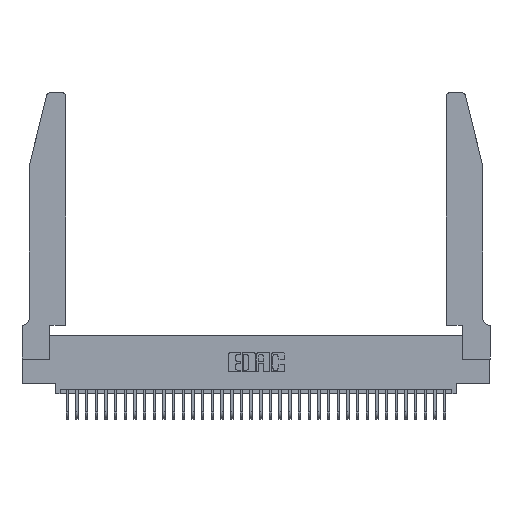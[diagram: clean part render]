
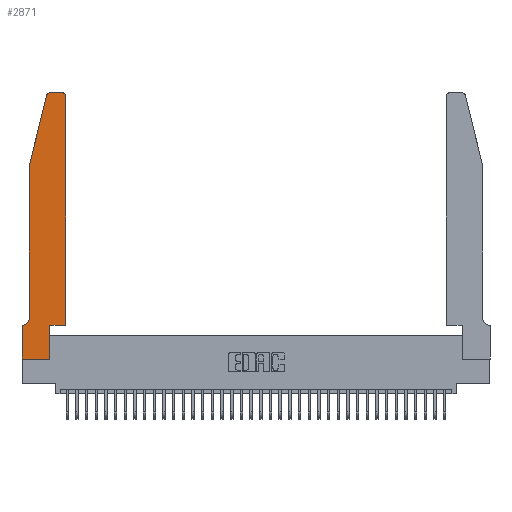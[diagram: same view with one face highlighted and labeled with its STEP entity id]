
A CAD part, top view. The second image highlights one B-rep face of the part: STEP entity #2871.
In plain terms, the highlighted planar face has unit normal (0, 0, 1).
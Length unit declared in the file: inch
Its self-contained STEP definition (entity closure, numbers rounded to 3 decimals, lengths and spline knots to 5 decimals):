
#1622 = EDGE_CURVE ( 'NONE', #17877, #11990, #17657, .T. ) ;
#1650 = CARTESIAN_POINT ( 'NONE',  ( 0., 0., 0.37 ) ) ;
#1932 = AXIS2_PLACEMENT_3D ( 'NONE', #25203, #11675, #30626 ) ;
#2622 = CARTESIAN_POINT ( 'NONE',  ( 0.0055, 0.35, 0.37 ) ) ;
#2848 = AXIS2_PLACEMENT_3D ( 'NONE', #14310, #33249, #17055 ) ;
#2871 = ADVANCED_FACE ( 'NONE', ( #5608 ), #8942, .T. ) ;
#3245 = ORIENTED_EDGE ( 'NONE', *, *, #9922, .T. ) ;
#4492 = ORIENTED_EDGE ( 'NONE', *, *, #1622, .T. ) ;
#5138 = EDGE_CURVE ( 'NONE', #32559, #6090, #13553, .T. ) ;
#5183 = VERTEX_POINT ( 'NONE', #2622 ) ;
#5518 = CARTESIAN_POINT ( 'NONE',  ( 0., 0., 0.37 ) ) ;
#5608 = FACE_OUTER_BOUND ( 'NONE', #26734, .T. ) ;
#6090 = VERTEX_POINT ( 'NONE', #24493 ) ;
#6145 = VERTEX_POINT ( 'NONE', #8455 ) ;
#6297 = VECTOR ( 'NONE', #32265, 39.37008 ) ;
#7257 = DIRECTION ( 'NONE',  ( 0., -1., 0. ) ) ;
#7397 = CARTESIAN_POINT ( 'NONE',  ( 0.4205, 2.72, 0.37 ) ) ;
#7553 = CARTESIAN_POINT ( 'NONE',  ( 0.2605, 2.75, 0.37 ) ) ;
#7961 = ORIENTED_EDGE ( 'NONE', *, *, #5138, .T. ) ;
#8039 = ORIENTED_EDGE ( 'NONE', *, *, #30061, .T. ) ;
#8318 = ORIENTED_EDGE ( 'NONE', *, *, #28478, .T. ) ;
#8455 = CARTESIAN_POINT ( 'NONE',  ( 0., 0.35, 0.37 ) ) ;
#8689 = CARTESIAN_POINT ( 'NONE',  ( 0.0755, 2., 0.37 ) ) ;
#8726 = ORIENTED_EDGE ( 'NONE', *, *, #23400, .T. ) ;
#8939 = ORIENTED_EDGE ( 'NONE', *, *, #12916, .T. ) ;
#8942 = PLANE ( 'NONE',  #1932 ) ;
#9538 = CARTESIAN_POINT ( 'NONE',  ( 0.2865, 0.35, 0.37 ) ) ;
#9587 = VECTOR ( 'NONE', #21124, 39.37008 ) ;
#9773 = DIRECTION ( 'NONE',  ( 0., 0., 1. ) ) ;
#9900 = VECTOR ( 'NONE', #33381, 39.37008 ) ;
#9922 = EDGE_CURVE ( 'NONE', #26077, #32559, #25986, .T. ) ;
#9949 = EDGE_CURVE ( 'NONE', #32544, #17877, #25138, .T. ) ;
#10133 = DIRECTION ( 'NONE',  ( 1., 0., 0. ) ) ;
#11533 = VECTOR ( 'NONE', #32969, 39.37008 ) ;
#11675 = DIRECTION ( 'NONE',  ( 0., 0., 1. ) ) ;
#11715 = CARTESIAN_POINT ( 'NONE',  ( 0.0755, 2., 0.37 ) ) ;
#11990 = VERTEX_POINT ( 'NONE', #26835 ) ;
#12029 = CARTESIAN_POINT ( 'NONE',  ( 0., 0., 0.37 ) ) ;
#12386 = DIRECTION ( 'NONE',  ( 0., 1., 0. ) ) ;
#12663 = VERTEX_POINT ( 'NONE', #34920 ) ;
#12916 = EDGE_CURVE ( 'NONE', #28007, #5183, #23666, .T. ) ;
#13274 = CARTESIAN_POINT ( 'NONE',  ( 0.2865, 0., 0.37 ) ) ;
#13553 = LINE ( 'NONE', #29552, #6297 ) ;
#13973 = CARTESIAN_POINT ( 'NONE',  ( 0.4205, 2.75, 0.37 ) ) ;
#14028 = AXIS2_PLACEMENT_3D ( 'NONE', #26025, #9773, #28753 ) ;
#14310 = CARTESIAN_POINT ( 'NONE',  ( 0.0055, 0.42, 0.37 ) ) ;
#15443 = LINE ( 'NONE', #11715, #9900 ) ;
#16721 = ORIENTED_EDGE ( 'NONE', *, *, #31541, .T. ) ;
#16870 = VERTEX_POINT ( 'NONE', #13973 ) ;
#17055 = DIRECTION ( 'NONE',  ( -1., 0., 0. ) ) ;
#17642 = CARTESIAN_POINT ( 'NONE',  ( 0.284, 2.75, 0.37 ) ) ;
#17657 = LINE ( 'NONE', #8689, #23170 ) ;
#17771 = CARTESIAN_POINT ( 'NONE',  ( 0.2865, 0.35, 0.37 ) ) ;
#17795 = VECTOR ( 'NONE', #20270, 39.37008 ) ;
#17877 = VERTEX_POINT ( 'NONE', #21547 ) ;
#18110 = LINE ( 'NONE', #22731, #31626 ) ;
#19560 = EDGE_CURVE ( 'NONE', #12663, #16870, #25507, .T. ) ;
#19749 = LINE ( 'NONE', #1650, #33234 ) ;
#20270 = DIRECTION ( 'NONE',  ( 1., 0., 0. ) ) ;
#20604 = ORIENTED_EDGE ( 'NONE', *, *, #27098, .T. ) ;
#21124 = DIRECTION ( 'NONE',  ( -1., 0., 0. ) ) ;
#21547 = CARTESIAN_POINT ( 'NONE',  ( 0.25487, 2.72718, 0.37 ) ) ;
#21554 = ORIENTED_EDGE ( 'NONE', *, *, #9949, .T. ) ;
#22118 = ORIENTED_EDGE ( 'NONE', *, *, #22577, .T. ) ;
#22577 = EDGE_CURVE ( 'NONE', #6090, #12663, #18110, .T. ) ;
#22731 = CARTESIAN_POINT ( 'NONE',  ( 0.4505, 0.35, 0.37 ) ) ;
#23170 = VECTOR ( 'NONE', #24954, 39.37008 ) ;
#23400 = EDGE_CURVE ( 'NONE', #6145, #27888, #19749, .T. ) ;
#23666 = CIRCLE ( 'NONE', #2848, 0.07 ) ;
#24493 = CARTESIAN_POINT ( 'NONE',  ( 0.4505, 0.35, 0.37 ) ) ;
#24954 = DIRECTION ( 'NONE',  ( -0.239, -0.971, 0. ) ) ;
#24987 = LINE ( 'NONE', #12029, #17795 ) ;
#25138 = CIRCLE ( 'NONE', #14028, 0.03 ) ;
#25140 = CARTESIAN_POINT ( 'NONE',  ( 0.0755, 0.42, 0.37 ) ) ;
#25203 = CARTESIAN_POINT ( 'NONE',  ( 0., 0.35, 0.37 ) ) ;
#25422 = DIRECTION ( 'NONE',  ( 0., 1., 0. ) ) ;
#25507 = CIRCLE ( 'NONE', #31262, 0.03 ) ;
#25986 = LINE ( 'NONE', #9538, #32315 ) ;
#26025 = CARTESIAN_POINT ( 'NONE',  ( 0.284, 2.72, 0.37 ) ) ;
#26077 = VERTEX_POINT ( 'NONE', #13274 ) ;
#26401 = DIRECTION ( 'NONE',  ( 0., 0., 1. ) ) ;
#26734 = EDGE_LOOP ( 'NONE', ( #8318, #21554, #4492, #8039, #8939, #16721, #8726, #20604, #3245, #7961, #22118, #27320 ) ) ;
#26835 = CARTESIAN_POINT ( 'NONE',  ( 0.0755, 2., 0.37 ) ) ;
#27098 = EDGE_CURVE ( 'NONE', #27888, #26077, #24987, .T. ) ;
#27320 = ORIENTED_EDGE ( 'NONE', *, *, #19560, .T. ) ;
#27888 = VERTEX_POINT ( 'NONE', #5518 ) ;
#28007 = VERTEX_POINT ( 'NONE', #25140 ) ;
#28478 = EDGE_CURVE ( 'NONE', #16870, #32544, #31216, .T. ) ;
#28753 = DIRECTION ( 'NONE',  ( 1., 0., 0. ) ) ;
#29552 = CARTESIAN_POINT ( 'NONE',  ( 0.4505, 0.35, 0.37 ) ) ;
#30061 = EDGE_CURVE ( 'NONE', #11990, #28007, #15443, .T. ) ;
#30259 = CARTESIAN_POINT ( 'NONE',  ( 0.0755, 0.35, 0.37 ) ) ;
#30626 = DIRECTION ( 'NONE',  ( 1., 0., 0. ) ) ;
#31216 = LINE ( 'NONE', #7553, #9587 ) ;
#31262 = AXIS2_PLACEMENT_3D ( 'NONE', #7397, #26401, #10133 ) ;
#31541 = EDGE_CURVE ( 'NONE', #5183, #6145, #33154, .T. ) ;
#31626 = VECTOR ( 'NONE', #25422, 39.37008 ) ;
#32265 = DIRECTION ( 'NONE',  ( 1., 0., 0. ) ) ;
#32315 = VECTOR ( 'NONE', #12386, 39.37008 ) ;
#32544 = VERTEX_POINT ( 'NONE', #17642 ) ;
#32559 = VERTEX_POINT ( 'NONE', #17771 ) ;
#32969 = DIRECTION ( 'NONE',  ( -1., 0., 0. ) ) ;
#33154 = LINE ( 'NONE', #30259, #11533 ) ;
#33234 = VECTOR ( 'NONE', #7257, 39.37008 ) ;
#33249 = DIRECTION ( 'NONE',  ( 0., 0., -1. ) ) ;
#33381 = DIRECTION ( 'NONE',  ( 0., -1., 0. ) ) ;
#34920 = CARTESIAN_POINT ( 'NONE',  ( 0.4505, 2.72, 0.37 ) ) ;
